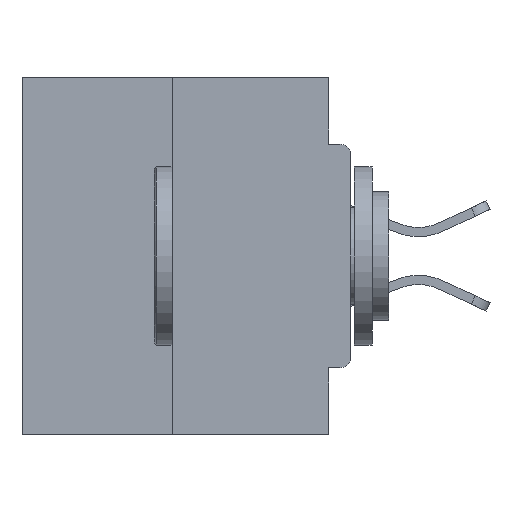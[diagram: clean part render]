
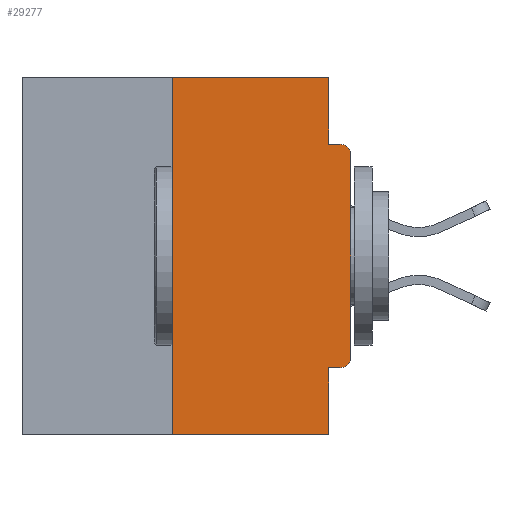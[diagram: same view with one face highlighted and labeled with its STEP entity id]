
A CAD part, left-side view. The second image highlights one B-rep face of the part: STEP entity #29277.
In plain terms, the highlighted planar face has unit normal (-1, 0, 0).
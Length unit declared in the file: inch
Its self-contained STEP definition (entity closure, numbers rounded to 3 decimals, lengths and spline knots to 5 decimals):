
#288 = PLANE ( 'NONE',  #27841 ) ;
#341 = CARTESIAN_POINT ( 'NONE',  ( 0., 0., -0.3915 ) ) ;
#746 = DIRECTION ( 'NONE',  ( 0., -1., 0. ) ) ;
#832 = CARTESIAN_POINT ( 'NONE',  ( 0., 0.015, -0.4065 ) ) ;
#1424 = CARTESIAN_POINT ( 'NONE',  ( 0., 0.25, 0. ) ) ;
#1536 = EDGE_CURVE ( 'NONE', #22819, #32970, #12042, .T. ) ;
#2600 = DIRECTION ( 'NONE',  ( 0., 0., -1. ) ) ;
#2621 = VECTOR ( 'NONE', #33303, 39.37008 ) ;
#3093 = VERTEX_POINT ( 'NONE', #341 ) ;
#3373 = VECTOR ( 'NONE', #14720, 39.37008 ) ;
#4112 = CARTESIAN_POINT ( 'NONE',  ( 0., 0., 0. ) ) ;
#4993 = LINE ( 'NONE', #1424, #3373 ) ;
#5216 = DIRECTION ( 'NONE',  ( 0., 1., 0. ) ) ;
#5256 = CARTESIAN_POINT ( 'NONE',  ( 0., 0.25, -0.5 ) ) ;
#5545 = VECTOR ( 'NONE', #14379, 39.37008 ) ;
#5633 = CARTESIAN_POINT ( 'NONE',  ( 0., 0.031, 0. ) ) ;
#5863 = EDGE_LOOP ( 'NONE', ( #24381, #28118, #12016, #12209, #14662, #22315, #29068, #9175, #11459, #7992 ) ) ;
#7030 = EDGE_CURVE ( 'NONE', #28810, #13752, #13029, .T. ) ;
#7514 = EDGE_CURVE ( 'NONE', #3093, #22819, #15031, .T. ) ;
#7635 = VERTEX_POINT ( 'NONE', #5256 ) ;
#7992 = ORIENTED_EDGE ( 'NONE', *, *, #15880, .F. ) ;
#8129 = CARTESIAN_POINT ( 'NONE',  ( 0., 0.031, -0.5 ) ) ;
#8308 = CARTESIAN_POINT ( 'NONE',  ( 0., 0.031, -0.4065 ) ) ;
#8354 = DIRECTION ( 'NONE',  ( 1., 0., 0. ) ) ;
#9052 = EDGE_CURVE ( 'NONE', #32549, #28197, #22691, .T. ) ;
#9175 = ORIENTED_EDGE ( 'NONE', *, *, #1536, .T. ) ;
#10919 = LINE ( 'NONE', #17818, #14610 ) ;
#10982 = CARTESIAN_POINT ( 'NONE',  ( 0., 0.46, 0. ) ) ;
#11124 = DIRECTION ( 'NONE',  ( 0., 0., -1. ) ) ;
#11459 = ORIENTED_EDGE ( 'NONE', *, *, #20785, .F. ) ;
#12016 = ORIENTED_EDGE ( 'NONE', *, *, #30756, .T. ) ;
#12042 = CIRCLE ( 'NONE', #20105, 0.015 ) ;
#12209 = ORIENTED_EDGE ( 'NONE', *, *, #15849, .F. ) ;
#12307 = DIRECTION ( 'NONE',  ( 0., 0., -1. ) ) ;
#13029 = LINE ( 'NONE', #10982, #26594 ) ;
#13558 = LINE ( 'NONE', #16542, #25038 ) ;
#13752 = VERTEX_POINT ( 'NONE', #21328 ) ;
#14162 = VERTEX_POINT ( 'NONE', #22896 ) ;
#14379 = DIRECTION ( 'NONE',  ( 0., 0., 1. ) ) ;
#14610 = VECTOR ( 'NONE', #23007, 39.37008 ) ;
#14662 = ORIENTED_EDGE ( 'NONE', *, *, #9052, .F. ) ;
#14720 = DIRECTION ( 'NONE',  ( 0., 0., 1. ) ) ;
#15031 = LINE ( 'NONE', #4112, #5545 ) ;
#15173 = CARTESIAN_POINT ( 'NONE',  ( 0., 0.015, -0.1085 ) ) ;
#15849 = EDGE_CURVE ( 'NONE', #28197, #18563, #10919, .T. ) ;
#15880 = EDGE_CURVE ( 'NONE', #13752, #14162, #24883, .T. ) ;
#16445 = CARTESIAN_POINT ( 'NONE',  ( 0., 0.015, -0.3915 ) ) ;
#16542 = CARTESIAN_POINT ( 'NONE',  ( 0., 0., -0.0935 ) ) ;
#16659 = CARTESIAN_POINT ( 'NONE',  ( 0., 0.25, 0. ) ) ;
#16660 = DIRECTION ( 'NONE',  ( -1., 0., 0. ) ) ;
#17243 = CARTESIAN_POINT ( 'NONE',  ( 0., 0.46, -0.5 ) ) ;
#17379 = EDGE_CURVE ( 'NONE', #7635, #28810, #4993, .T. ) ;
#17509 = AXIS2_PLACEMENT_3D ( 'NONE', #16445, #16660, #19977 ) ;
#17818 = CARTESIAN_POINT ( 'NONE',  ( 0., 0.031, -0.5 ) ) ;
#18563 = VERTEX_POINT ( 'NONE', #8129 ) ;
#19062 = CARTESIAN_POINT ( 'NONE',  ( 0., 0.015, -0.0935 ) ) ;
#19977 = DIRECTION ( 'NONE',  ( 0., 0., -1. ) ) ;
#20105 = AXIS2_PLACEMENT_3D ( 'NONE', #15173, #25401, #12307 ) ;
#20785 = EDGE_CURVE ( 'NONE', #14162, #32970, #13558, .T. ) ;
#20968 = CARTESIAN_POINT ( 'NONE',  ( 0., 0., -0.4065 ) ) ;
#21328 = CARTESIAN_POINT ( 'NONE',  ( 0., 0.031, 0. ) ) ;
#22315 = ORIENTED_EDGE ( 'NONE', *, *, #32088, .T. ) ;
#22691 = LINE ( 'NONE', #20968, #23139 ) ;
#22819 = VERTEX_POINT ( 'NONE', #32301 ) ;
#22896 = CARTESIAN_POINT ( 'NONE',  ( 0., 0.031, -0.0935 ) ) ;
#23007 = DIRECTION ( 'NONE',  ( 0., 0., -1. ) ) ;
#23139 = VECTOR ( 'NONE', #5216, 39.37008 ) ;
#23643 = VECTOR ( 'NONE', #2600, 39.37008 ) ;
#24381 = ORIENTED_EDGE ( 'NONE', *, *, #7030, .F. ) ;
#24883 = LINE ( 'NONE', #5633, #23643 ) ;
#25038 = VECTOR ( 'NONE', #746, 39.37008 ) ;
#25293 = CIRCLE ( 'NONE', #17509, 0.015 ) ;
#25401 = DIRECTION ( 'NONE',  ( -1., 0., 0. ) ) ;
#26099 = LINE ( 'NONE', #17243, #2621 ) ;
#26594 = VECTOR ( 'NONE', #32183, 39.37008 ) ;
#27485 = FACE_OUTER_BOUND ( 'NONE', #5863, .T. ) ;
#27841 = AXIS2_PLACEMENT_3D ( 'NONE', #29726, #8354, #11124 ) ;
#28118 = ORIENTED_EDGE ( 'NONE', *, *, #17379, .F. ) ;
#28197 = VERTEX_POINT ( 'NONE', #8308 ) ;
#28810 = VERTEX_POINT ( 'NONE', #16659 ) ;
#29068 = ORIENTED_EDGE ( 'NONE', *, *, #7514, .T. ) ;
#29277 = ADVANCED_FACE ( 'NONE', ( #27485 ), #288, .F. ) ;
#29726 = CARTESIAN_POINT ( 'NONE',  ( 0., 0.46, 0. ) ) ;
#30756 = EDGE_CURVE ( 'NONE', #7635, #18563, #26099, .T. ) ;
#32088 = EDGE_CURVE ( 'NONE', #32549, #3093, #25293, .T. ) ;
#32183 = DIRECTION ( 'NONE',  ( 0., -1., 0. ) ) ;
#32301 = CARTESIAN_POINT ( 'NONE',  ( 0., 0., -0.1085 ) ) ;
#32549 = VERTEX_POINT ( 'NONE', #832 ) ;
#32970 = VERTEX_POINT ( 'NONE', #19062 ) ;
#33303 = DIRECTION ( 'NONE',  ( 0., -1., 0. ) ) ;
